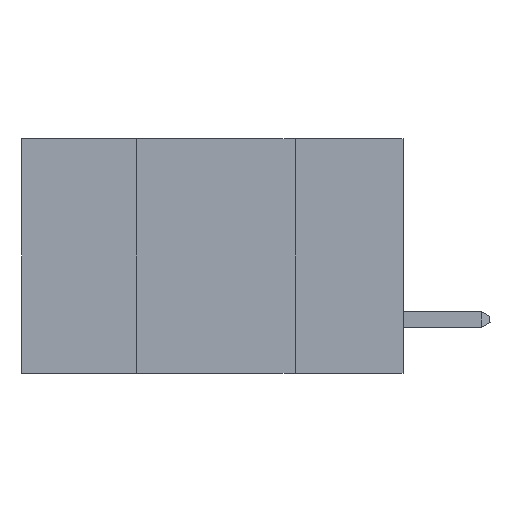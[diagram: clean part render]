
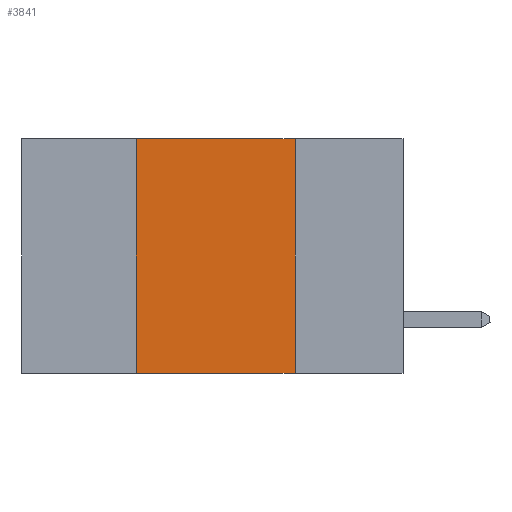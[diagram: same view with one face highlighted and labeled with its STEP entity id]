
A CAD part, left-side view. The second image highlights one B-rep face of the part: STEP entity #3841.
In plain terms, the highlighted planar face has unit normal (-1, 0, 0).
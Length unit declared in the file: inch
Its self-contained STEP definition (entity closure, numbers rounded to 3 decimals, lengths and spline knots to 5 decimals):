
#497 = EDGE_CURVE ( 'NONE', #8960, #12456, #10306, .T. ) ;
#654 = CARTESIAN_POINT ( 'NONE',  ( 0., 0.6, -0.37 ) ) ;
#1306 = EDGE_CURVE ( 'NONE', #12456, #6249, #12092, .T. ) ;
#1345 = LINE ( 'NONE', #654, #3336 ) ;
#3252 = CARTESIAN_POINT ( 'NONE',  ( 0., 0.17, -0.37 ) ) ;
#3336 = VECTOR ( 'NONE', #7579, 39.37008 ) ;
#3617 = DIRECTION ( 'NONE',  ( 0., 0., 1. ) ) ;
#3718 = DIRECTION ( 'NONE',  ( 1., 0., 0. ) ) ;
#3841 = ADVANCED_FACE ( 'NONE', ( #9668 ), #5499, .F. ) ;
#3901 = CARTESIAN_POINT ( 'NONE',  ( 0., 0.42, 0. ) ) ;
#4840 = DIRECTION ( 'NONE',  ( 0., 0., -1. ) ) ;
#5499 = PLANE ( 'NONE',  #6802 ) ;
#5563 = ORIENTED_EDGE ( 'NONE', *, *, #1306, .F. ) ;
#6249 = VERTEX_POINT ( 'NONE', #3252 ) ;
#6403 = VERTEX_POINT ( 'NONE', #11580 ) ;
#6802 = AXIS2_PLACEMENT_3D ( 'NONE', #13816, #3718, #4840 ) ;
#7579 = DIRECTION ( 'NONE',  ( 0., -1., 0. ) ) ;
#8032 = ORIENTED_EDGE ( 'NONE', *, *, #11958, .T. ) ;
#8398 = ORIENTED_EDGE ( 'NONE', *, *, #14868, .F. ) ;
#8444 = ORIENTED_EDGE ( 'NONE', *, *, #497, .F. ) ;
#8960 = VERTEX_POINT ( 'NONE', #3901 ) ;
#9668 = FACE_OUTER_BOUND ( 'NONE', #11316, .T. ) ;
#9972 = CARTESIAN_POINT ( 'NONE',  ( 0., 0.17, 0. ) ) ;
#10306 = LINE ( 'NONE', #13849, #12313 ) ;
#10734 = CARTESIAN_POINT ( 'NONE',  ( 0., 0.42, 0. ) ) ;
#10833 = VECTOR ( 'NONE', #11094, 39.37008 ) ;
#11094 = DIRECTION ( 'NONE',  ( 0., 0., -1. ) ) ;
#11316 = EDGE_LOOP ( 'NONE', ( #5563, #8444, #8398, #8032 ) ) ;
#11580 = CARTESIAN_POINT ( 'NONE',  ( 0., 0.42, -0.37 ) ) ;
#11958 = EDGE_CURVE ( 'NONE', #6403, #6249, #1345, .T. ) ;
#12092 = LINE ( 'NONE', #9972, #10833 ) ;
#12313 = VECTOR ( 'NONE', #12717, 39.37008 ) ;
#12456 = VERTEX_POINT ( 'NONE', #13378 ) ;
#12717 = DIRECTION ( 'NONE',  ( 0., -1., 0. ) ) ;
#13050 = LINE ( 'NONE', #10734, #13773 ) ;
#13378 = CARTESIAN_POINT ( 'NONE',  ( 0., 0.17, 0. ) ) ;
#13773 = VECTOR ( 'NONE', #3617, 39.37008 ) ;
#13816 = CARTESIAN_POINT ( 'NONE',  ( 0., 0.6, 0. ) ) ;
#13849 = CARTESIAN_POINT ( 'NONE',  ( 0., 0.6, 0. ) ) ;
#14868 = EDGE_CURVE ( 'NONE', #6403, #8960, #13050, .T. ) ;
